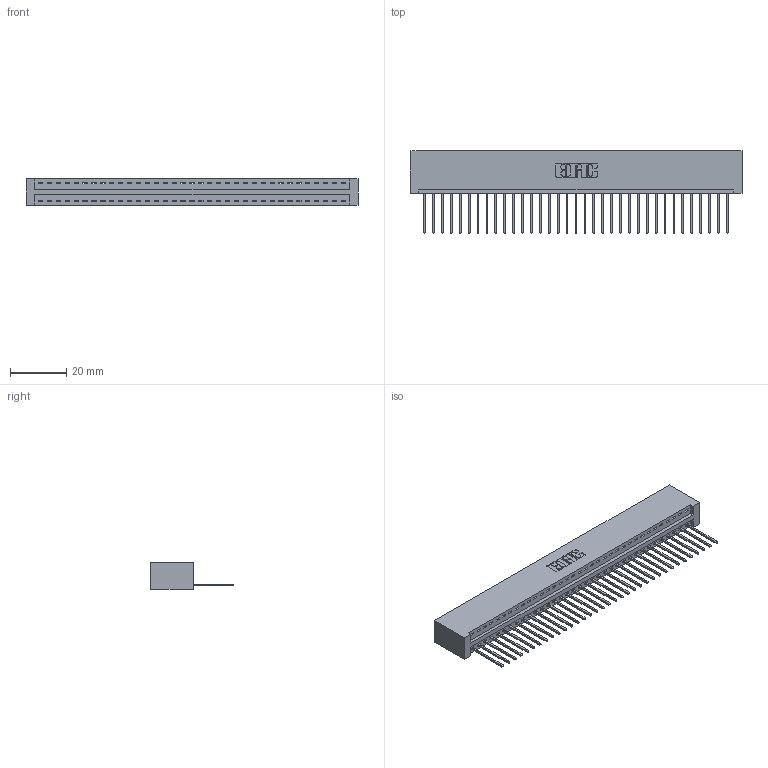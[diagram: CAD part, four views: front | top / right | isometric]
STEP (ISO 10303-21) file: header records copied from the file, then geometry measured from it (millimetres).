
FILE_DESCRIPTION (( 'STEP AP203' ), '1' );
FILE_NAME ('346-035-540-101.STEP', '2018-08-24T00:10:04', ( '' ), ( '' ), 'SwSTEP 2.0', 'SolidWorks 2016', '' );
FILE_SCHEMA (( 'CONFIG_CONTROL_DESIGN' ));
Length unit declared in the file: inch
Products named in the file (3): 346 Part_No Mounting Lugs; 345-292-001_345-293-140; 346-035-540-101
Assembly tree (36 placements, depth 2):
  346-035-540-101
    346 Part_No Mounting Lugs
    345-292-001_345-293-140  x35
Bounding box: 118.36 x 29.46 x 9.4 mm (x, y, z)
Volume: 11878.6 mm3; surface area: 15192.3 mm2
Topology: 36 solids, 36 shells, 2144 faces, 6465 edges, 4262 vertices
Faces by surface type: plane 1472, cylinder 672
Entity records: 22405 total; most frequent: CARTESIAN_POINT 3849, ORIENTED_EDGE 3818, DIRECTION 3399, EDGE_CURVE 1909, VECTOR 1645, LINE 1645, VERTEX_POINT 1270, AXIS2_PLACEMENT_3D 877
